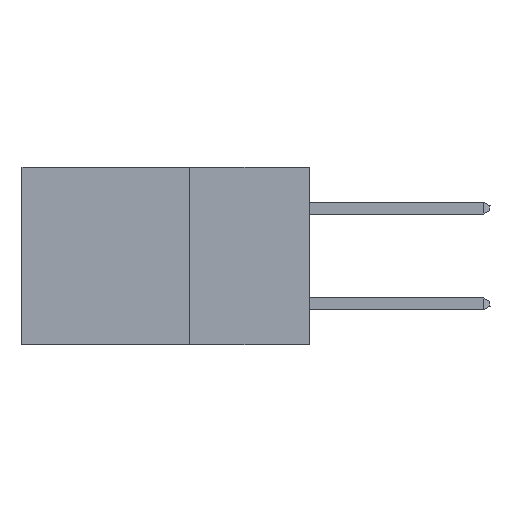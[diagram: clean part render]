
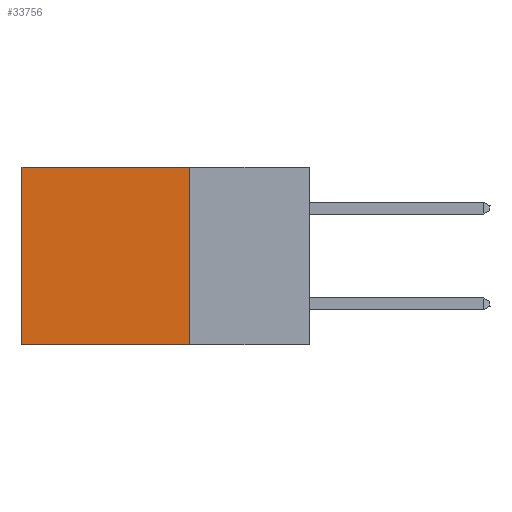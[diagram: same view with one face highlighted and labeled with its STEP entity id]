
A CAD part, left-side view. The second image highlights one B-rep face of the part: STEP entity #33756.
In plain terms, the highlighted planar face has unit normal (-1, 0, 0).
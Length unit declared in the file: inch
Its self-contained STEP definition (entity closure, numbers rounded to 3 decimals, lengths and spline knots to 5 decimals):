
#1859 = EDGE_CURVE ( 'NONE', #3204, #38074, #26656, .T. ) ;
#1875 = EDGE_CURVE ( 'NONE', #38074, #9585, #5304, .T. ) ;
#2883 = CARTESIAN_POINT ( 'NONE',  ( 0.2875, 0.25, 0. ) ) ;
#3204 = VERTEX_POINT ( 'NONE', #33930 ) ;
#3666 = CARTESIAN_POINT ( 'NONE',  ( 0.2875, 0.6, -0.37 ) ) ;
#3672 = DIRECTION ( 'NONE',  ( 0., 0., -1. ) ) ;
#3804 = VECTOR ( 'NONE', #42861, 39.37008 ) ;
#5304 = LINE ( 'NONE', #13168, #8022 ) ;
#7276 = VERTEX_POINT ( 'NONE', #28464 ) ;
#7586 = PLANE ( 'NONE',  #28550 ) ;
#8022 = VECTOR ( 'NONE', #13459, 39.37008 ) ;
#9585 = VERTEX_POINT ( 'NONE', #3666 ) ;
#11138 = ORIENTED_EDGE ( 'NONE', *, *, #32196, .F. ) ;
#13168 = CARTESIAN_POINT ( 'NONE',  ( 0.2875, 0.6, 0. ) ) ;
#13459 = DIRECTION ( 'NONE',  ( 0., 0., -1. ) ) ;
#14793 = EDGE_LOOP ( 'NONE', ( #21120, #11138, #28994, #43431 ) ) ;
#15347 = CARTESIAN_POINT ( 'NONE',  ( 0.2875, 0.25, -0.37 ) ) ;
#21120 = ORIENTED_EDGE ( 'NONE', *, *, #1875, .T. ) ;
#22958 = VECTOR ( 'NONE', #26691, 39.37008 ) ;
#25692 = EDGE_CURVE ( 'NONE', #3204, #7276, #35711, .T. ) ;
#26656 = LINE ( 'NONE', #2883, #22958 ) ;
#26691 = DIRECTION ( 'NONE',  ( 0., 1., 0. ) ) ;
#27972 = CARTESIAN_POINT ( 'NONE',  ( 0.2875, 0.6, 0. ) ) ;
#28464 = CARTESIAN_POINT ( 'NONE',  ( 0.2875, 0.25, -0.37 ) ) ;
#28550 = AXIS2_PLACEMENT_3D ( 'NONE', #34596, #40986, #3672 ) ;
#28711 = FACE_OUTER_BOUND ( 'NONE', #14793, .T. ) ;
#28994 = ORIENTED_EDGE ( 'NONE', *, *, #25692, .F. ) ;
#30939 = VECTOR ( 'NONE', #39073, 39.37008 ) ;
#32002 = LINE ( 'NONE', #15347, #30939 ) ;
#32196 = EDGE_CURVE ( 'NONE', #7276, #9585, #32002, .T. ) ;
#32613 = CARTESIAN_POINT ( 'NONE',  ( 0.2875, 0.25, 0. ) ) ;
#33756 = ADVANCED_FACE ( 'NONE', ( #28711 ), #7586, .F. ) ;
#33930 = CARTESIAN_POINT ( 'NONE',  ( 0.2875, 0.25, 0. ) ) ;
#34596 = CARTESIAN_POINT ( 'NONE',  ( 0.2875, 0.25, 0. ) ) ;
#35711 = LINE ( 'NONE', #32613, #3804 ) ;
#38074 = VERTEX_POINT ( 'NONE', #27972 ) ;
#39073 = DIRECTION ( 'NONE',  ( 0., 1., 0. ) ) ;
#40986 = DIRECTION ( 'NONE',  ( 1., 0., 0. ) ) ;
#42861 = DIRECTION ( 'NONE',  ( 0., 0., -1. ) ) ;
#43431 = ORIENTED_EDGE ( 'NONE', *, *, #1859, .T. ) ;
